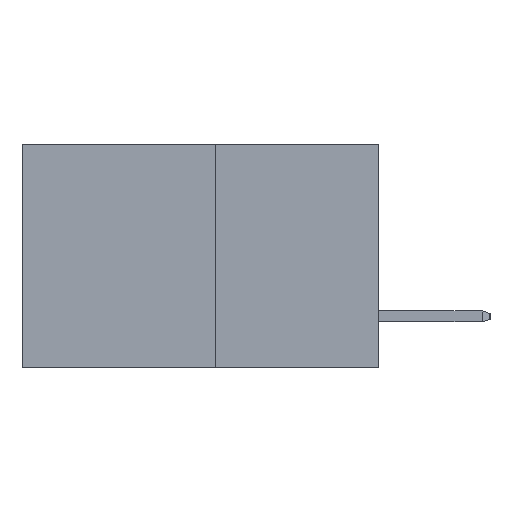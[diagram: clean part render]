
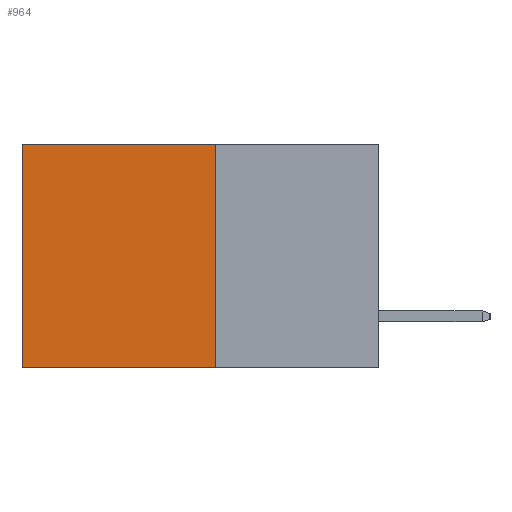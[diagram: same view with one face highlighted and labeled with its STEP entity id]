
A CAD part, left-side view. The second image highlights one B-rep face of the part: STEP entity #964.
In plain terms, the highlighted planar face has unit normal (-1, 0, 0).
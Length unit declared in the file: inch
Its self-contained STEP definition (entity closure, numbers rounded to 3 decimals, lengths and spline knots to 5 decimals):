
#251 = VECTOR ( 'NONE', #10661, 39.37008 ) ;
#590 = CARTESIAN_POINT ( 'NONE',  ( 0.277, 0.27, 0. ) ) ;
#964 = ADVANCED_FACE ( 'NONE', ( #7211 ), #10740, .F. ) ;
#1005 = VECTOR ( 'NONE', #11837, 39.37008 ) ;
#1520 = EDGE_CURVE ( 'NONE', #3502, #6108, #8856, .T. ) ;
#1979 = DIRECTION ( 'NONE',  ( 0., 1., 0. ) ) ;
#2018 = EDGE_CURVE ( 'NONE', #3502, #8242, #2852, .T. ) ;
#2565 = DIRECTION ( 'NONE',  ( 1., 0., 0. ) ) ;
#2592 = DIRECTION ( 'NONE',  ( 0., 0., -1. ) ) ;
#2674 = AXIS2_PLACEMENT_3D ( 'NONE', #11244, #2565, #2592 ) ;
#2784 = ORIENTED_EDGE ( 'NONE', *, *, #1520, .F. ) ;
#2852 = LINE ( 'NONE', #10687, #251 ) ;
#3502 = VERTEX_POINT ( 'NONE', #590 ) ;
#3838 = CARTESIAN_POINT ( 'NONE',  ( 0.277, 0.27, -0.37 ) ) ;
#4175 = LINE ( 'NONE', #6183, #1005 ) ;
#6108 = VERTEX_POINT ( 'NONE', #3838 ) ;
#6183 = CARTESIAN_POINT ( 'NONE',  ( 0.277, 0.59, -0.37 ) ) ;
#6558 = VERTEX_POINT ( 'NONE', #11123 ) ;
#6576 = VECTOR ( 'NONE', #1979, 39.37008 ) ;
#6864 = EDGE_LOOP ( 'NONE', ( #9810, #12270, #2784, #10555 ) ) ;
#7211 = FACE_OUTER_BOUND ( 'NONE', #6864, .T. ) ;
#7569 = EDGE_CURVE ( 'NONE', #6108, #6558, #8234, .T. ) ;
#8234 = LINE ( 'NONE', #9620, #6576 ) ;
#8242 = VERTEX_POINT ( 'NONE', #9650 ) ;
#8517 = EDGE_CURVE ( 'NONE', #8242, #6558, #4175, .T. ) ;
#8565 = VECTOR ( 'NONE', #8665, 39.37008 ) ;
#8665 = DIRECTION ( 'NONE',  ( 0., 0., -1. ) ) ;
#8856 = LINE ( 'NONE', #9951, #8565 ) ;
#9620 = CARTESIAN_POINT ( 'NONE',  ( 0.277, 0.27, -0.37 ) ) ;
#9650 = CARTESIAN_POINT ( 'NONE',  ( 0.277, 0.59, 0. ) ) ;
#9810 = ORIENTED_EDGE ( 'NONE', *, *, #8517, .T. ) ;
#9951 = CARTESIAN_POINT ( 'NONE',  ( 0.277, 0.27, -0.37 ) ) ;
#10555 = ORIENTED_EDGE ( 'NONE', *, *, #2018, .T. ) ;
#10661 = DIRECTION ( 'NONE',  ( 0., 1., 0. ) ) ;
#10687 = CARTESIAN_POINT ( 'NONE',  ( 0.277, 0.27, 0. ) ) ;
#10740 = PLANE ( 'NONE',  #2674 ) ;
#11123 = CARTESIAN_POINT ( 'NONE',  ( 0.277, 0.59, -0.37 ) ) ;
#11244 = CARTESIAN_POINT ( 'NONE',  ( 0.277, 0.27, -0.37 ) ) ;
#11837 = DIRECTION ( 'NONE',  ( 0., 0., -1. ) ) ;
#12270 = ORIENTED_EDGE ( 'NONE', *, *, #7569, .F. ) ;
